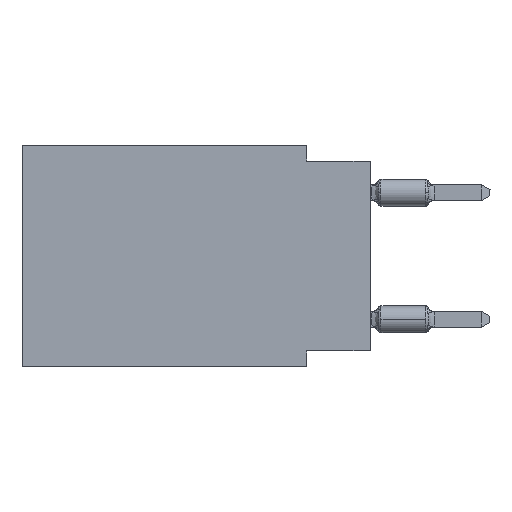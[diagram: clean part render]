
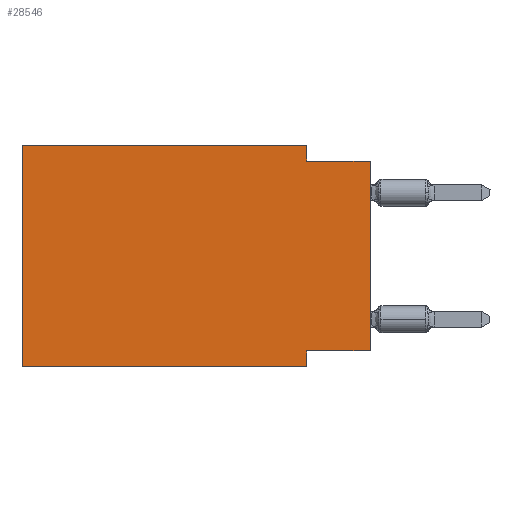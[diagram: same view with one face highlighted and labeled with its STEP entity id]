
A CAD part, left-side view. The second image highlights one B-rep face of the part: STEP entity #28546.
In plain terms, the highlighted planar face has unit normal (-1, 0, 0).
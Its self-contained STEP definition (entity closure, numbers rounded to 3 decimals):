
#331 = ORIENTED_EDGE ( 'NONE', *, *, #5182, .F. ) ;
#849 = VERTEX_POINT ( 'NONE', #44111 ) ;
#943 = EDGE_CURVE ( 'NONE', #6800, #42834, #37728, .T. ) ;
#1651 = LINE ( 'NONE', #12919, #21604 ) ;
#1958 = ORIENTED_EDGE ( 'NONE', *, *, #31941, .F. ) ;
#2029 = LINE ( 'NONE', #16693, #11150 ) ;
#3432 = ORIENTED_EDGE ( 'NONE', *, *, #37879, .F. ) ;
#4779 = LINE ( 'NONE', #27772, #43009 ) ;
#5182 = EDGE_CURVE ( 'NONE', #45849, #849, #20310, .T. ) ;
#5732 = VERTEX_POINT ( 'NONE', #9770 ) ;
#6684 = VECTOR ( 'NONE', #39734, 1000. ) ;
#6800 = VERTEX_POINT ( 'NONE', #16439 ) ;
#9770 = CARTESIAN_POINT ( 'NONE',  ( 0., 2.54, 0. ) ) ;
#10402 = CARTESIAN_POINT ( 'NONE',  ( 0., 0., 0. ) ) ;
#11150 = VECTOR ( 'NONE', #16456, 1000. ) ;
#12919 = CARTESIAN_POINT ( 'NONE',  ( 0., 0., -0.635 ) ) ;
#14150 = VERTEX_POINT ( 'NONE', #48348 ) ;
#16124 = ORIENTED_EDGE ( 'NONE', *, *, #21525, .F. ) ;
#16252 = CARTESIAN_POINT ( 'NONE',  ( 0., 2.54, -8.89 ) ) ;
#16426 = CARTESIAN_POINT ( 'NONE',  ( 0., 2.54, -8.89 ) ) ;
#16439 = CARTESIAN_POINT ( 'NONE',  ( 0., 2.54, -8.255 ) ) ;
#16456 = DIRECTION ( 'NONE',  ( 0., -1., 0. ) ) ;
#16693 = CARTESIAN_POINT ( 'NONE',  ( 0., 13.97, 0. ) ) ;
#17461 = DIRECTION ( 'NONE',  ( 0., 0., -1. ) ) ;
#17710 = PLANE ( 'NONE',  #28342 ) ;
#17832 = CARTESIAN_POINT ( 'NONE',  ( 0., 2.54, -0.635 ) ) ;
#19958 = CARTESIAN_POINT ( 'NONE',  ( 0., 13.97, -8.89 ) ) ;
#20310 = LINE ( 'NONE', #34740, #33545 ) ;
#21525 = EDGE_CURVE ( 'NONE', #44223, #6800, #4779, .T. ) ;
#21604 = VECTOR ( 'NONE', #30754, 1000. ) ;
#22648 = VERTEX_POINT ( 'NONE', #17832 ) ;
#23308 = DIRECTION ( 'NONE',  ( 0., 0., -1. ) ) ;
#23402 = DIRECTION ( 'NONE',  ( 0., -1., 0. ) ) ;
#24373 = ORIENTED_EDGE ( 'NONE', *, *, #26611, .F. ) ;
#24578 = VECTOR ( 'NONE', #25303, 1000. ) ;
#25303 = DIRECTION ( 'NONE',  ( 0., 0., 1. ) ) ;
#26160 = EDGE_CURVE ( 'NONE', #45849, #42834, #45664, .T. ) ;
#26611 = EDGE_CURVE ( 'NONE', #849, #5732, #2029, .T. ) ;
#27376 = EDGE_LOOP ( 'NONE', ( #37162, #1958, #3432, #24373, #331, #33466, #46304, #16124 ) ) ;
#27772 = CARTESIAN_POINT ( 'NONE',  ( 0., 0., -8.255 ) ) ;
#27927 = VECTOR ( 'NONE', #23308, 1000. ) ;
#28342 = AXIS2_PLACEMENT_3D ( 'NONE', #29423, #44335, #17461 ) ;
#28546 = ADVANCED_FACE ( 'NONE', ( #39699 ), #17710, .F. ) ;
#29423 = CARTESIAN_POINT ( 'NONE',  ( 0., 13.97, 0. ) ) ;
#30750 = CARTESIAN_POINT ( 'NONE',  ( 0., 13.97, -8.89 ) ) ;
#30754 = DIRECTION ( 'NONE',  ( 0., -1., 0. ) ) ;
#31323 = DIRECTION ( 'NONE',  ( 0., 0., 1. ) ) ;
#31941 = EDGE_CURVE ( 'NONE', #22648, #14150, #1651, .T. ) ;
#33466 = ORIENTED_EDGE ( 'NONE', *, *, #26160, .T. ) ;
#33545 = VECTOR ( 'NONE', #31323, 1000. ) ;
#34740 = CARTESIAN_POINT ( 'NONE',  ( 0., 13.97, 0. ) ) ;
#34929 = LINE ( 'NONE', #42509, #6684 ) ;
#37162 = ORIENTED_EDGE ( 'NONE', *, *, #44159, .T. ) ;
#37728 = LINE ( 'NONE', #16252, #27927 ) ;
#37879 = EDGE_CURVE ( 'NONE', #5732, #22648, #34929, .T. ) ;
#39000 = DIRECTION ( 'NONE',  ( 0., 1., 0. ) ) ;
#39699 = FACE_OUTER_BOUND ( 'NONE', #27376, .T. ) ;
#39734 = DIRECTION ( 'NONE',  ( 0., 0., -1. ) ) ;
#42509 = CARTESIAN_POINT ( 'NONE',  ( 0., 2.54, 0. ) ) ;
#42834 = VERTEX_POINT ( 'NONE', #16426 ) ;
#43009 = VECTOR ( 'NONE', #39000, 1000. ) ;
#43858 = LINE ( 'NONE', #10402, #24578 ) ;
#44111 = CARTESIAN_POINT ( 'NONE',  ( 0., 13.97, 0. ) ) ;
#44159 = EDGE_CURVE ( 'NONE', #44223, #14150, #43858, .T. ) ;
#44223 = VERTEX_POINT ( 'NONE', #45564 ) ;
#44335 = DIRECTION ( 'NONE',  ( 1., 0., 0. ) ) ;
#44662 = VECTOR ( 'NONE', #23402, 1000. ) ;
#45564 = CARTESIAN_POINT ( 'NONE',  ( 0., 0., -8.255 ) ) ;
#45664 = LINE ( 'NONE', #30750, #44662 ) ;
#45849 = VERTEX_POINT ( 'NONE', #19958 ) ;
#46304 = ORIENTED_EDGE ( 'NONE', *, *, #943, .F. ) ;
#48348 = CARTESIAN_POINT ( 'NONE',  ( 0., 0., -0.635 ) ) ;
